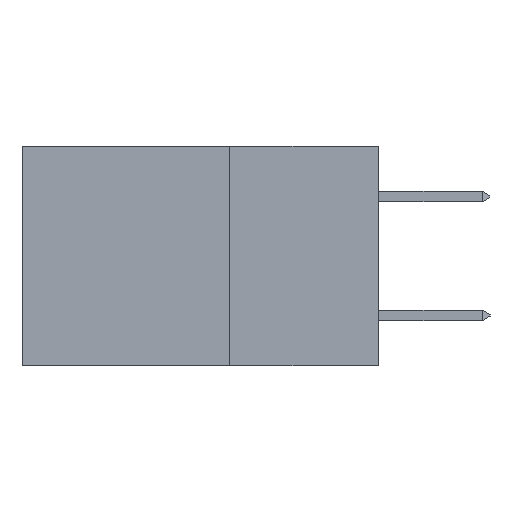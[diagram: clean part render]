
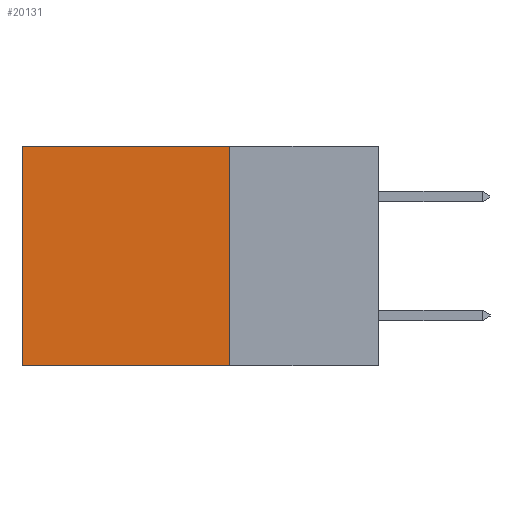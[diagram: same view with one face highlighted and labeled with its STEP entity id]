
A CAD part, left-side view. The second image highlights one B-rep face of the part: STEP entity #20131.
In plain terms, the highlighted planar face has unit normal (-1, 0, 0).
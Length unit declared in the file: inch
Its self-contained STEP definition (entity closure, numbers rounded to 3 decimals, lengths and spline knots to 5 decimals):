
#735 = VECTOR ( 'NONE', #16645, 39.37008 ) ;
#1387 = VECTOR ( 'NONE', #19331, 39.37008 ) ;
#1562 = CARTESIAN_POINT ( 'NONE',  ( 0.2615, 0.25, 0. ) ) ;
#3304 = LINE ( 'NONE', #22193, #23545 ) ;
#3438 = ORIENTED_EDGE ( 'NONE', *, *, #3997, .T. ) ;
#3997 = EDGE_CURVE ( 'NONE', #15244, #21069, #10964, .T. ) ;
#5366 = EDGE_CURVE ( 'NONE', #21069, #5853, #10876, .T. ) ;
#5521 = EDGE_CURVE ( 'NONE', #13756, #5853, #7842, .T. ) ;
#5853 = VERTEX_POINT ( 'NONE', #11785 ) ;
#6502 = PLANE ( 'NONE',  #8663 ) ;
#6780 = CARTESIAN_POINT ( 'NONE',  ( 0.2615, 0.25, -0.37 ) ) ;
#7842 = LINE ( 'NONE', #14978, #16823 ) ;
#8419 = DIRECTION ( 'NONE',  ( 1., 0., 0. ) ) ;
#8663 = AXIS2_PLACEMENT_3D ( 'NONE', #19841, #8419, #21747 ) ;
#10780 = ORIENTED_EDGE ( 'NONE', *, *, #5366, .T. ) ;
#10816 = DIRECTION ( 'NONE',  ( 0., 0., -1. ) ) ;
#10876 = LINE ( 'NONE', #16853, #735 ) ;
#10898 = EDGE_LOOP ( 'NONE', ( #10780, #13764, #18240, #3438 ) ) ;
#10964 = LINE ( 'NONE', #19542, #1387 ) ;
#11785 = CARTESIAN_POINT ( 'NONE',  ( 0.2615, 0.6, -0.37 ) ) ;
#13756 = VERTEX_POINT ( 'NONE', #6780 ) ;
#13764 = ORIENTED_EDGE ( 'NONE', *, *, #5521, .F. ) ;
#14978 = CARTESIAN_POINT ( 'NONE',  ( 0.2615, 0.25, -0.37 ) ) ;
#15151 = DIRECTION ( 'NONE',  ( 0., 1., 0. ) ) ;
#15244 = VERTEX_POINT ( 'NONE', #1562 ) ;
#16645 = DIRECTION ( 'NONE',  ( 0., 0., -1. ) ) ;
#16823 = VECTOR ( 'NONE', #15151, 39.37008 ) ;
#16853 = CARTESIAN_POINT ( 'NONE',  ( 0.2615, 0.6, -0.37 ) ) ;
#18240 = ORIENTED_EDGE ( 'NONE', *, *, #18287, .F. ) ;
#18287 = EDGE_CURVE ( 'NONE', #15244, #13756, #3304, .T. ) ;
#19331 = DIRECTION ( 'NONE',  ( 0., 1., 0. ) ) ;
#19542 = CARTESIAN_POINT ( 'NONE',  ( 0.2615, 0.25, 0. ) ) ;
#19841 = CARTESIAN_POINT ( 'NONE',  ( 0.2615, 0.25, -0.37 ) ) ;
#20131 = ADVANCED_FACE ( 'NONE', ( #21688 ), #6502, .F. ) ;
#21069 = VERTEX_POINT ( 'NONE', #24424 ) ;
#21688 = FACE_OUTER_BOUND ( 'NONE', #10898, .T. ) ;
#21747 = DIRECTION ( 'NONE',  ( 0., 0., -1. ) ) ;
#22193 = CARTESIAN_POINT ( 'NONE',  ( 0.2615, 0.25, -0.37 ) ) ;
#23545 = VECTOR ( 'NONE', #10816, 39.37008 ) ;
#24424 = CARTESIAN_POINT ( 'NONE',  ( 0.2615, 0.6, 0. ) ) ;
